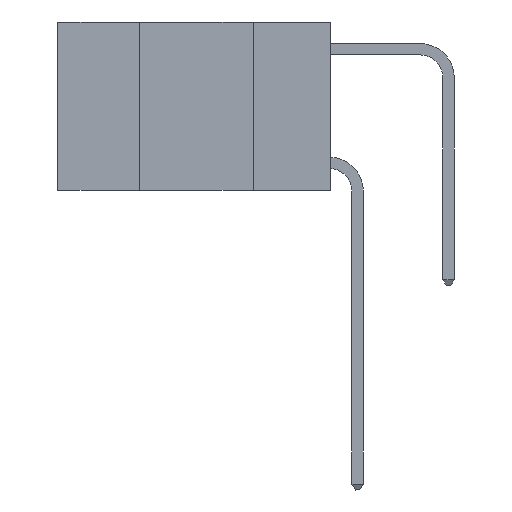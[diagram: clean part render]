
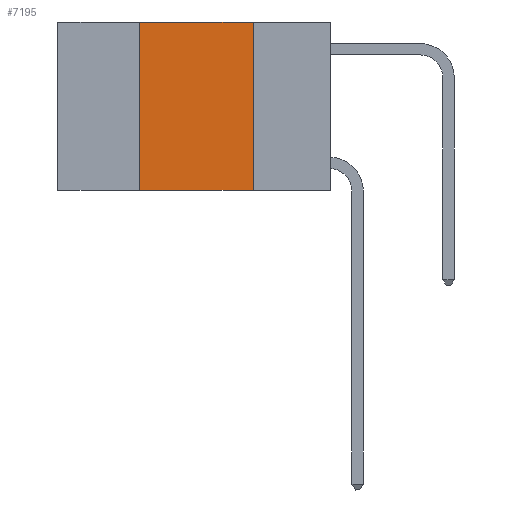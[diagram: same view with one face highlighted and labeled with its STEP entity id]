
A CAD part, left-side view. The second image highlights one B-rep face of the part: STEP entity #7195.
In plain terms, the highlighted planar face has unit normal (-1, 0, 0).
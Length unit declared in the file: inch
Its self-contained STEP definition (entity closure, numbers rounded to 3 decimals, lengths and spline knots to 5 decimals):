
#282 = CARTESIAN_POINT ( 'NONE',  ( 0., 0.6, 0. ) ) ;
#841 = VECTOR ( 'NONE', #5744, 39.37008 ) ;
#2904 = CARTESIAN_POINT ( 'NONE',  ( 0., 0.17, 0. ) ) ;
#2924 = CARTESIAN_POINT ( 'NONE',  ( 0., 0.6, 0. ) ) ;
#3123 = DIRECTION ( 'NONE',  ( 0., -1., 0. ) ) ;
#3323 = DIRECTION ( 'NONE',  ( 1., 0., 0. ) ) ;
#3525 = CARTESIAN_POINT ( 'NONE',  ( 0., 0.17, -0.37 ) ) ;
#3962 = CARTESIAN_POINT ( 'NONE',  ( 0., 0.42, -0.37 ) ) ;
#3967 = FACE_OUTER_BOUND ( 'NONE', #4237, .T. ) ;
#4157 = CARTESIAN_POINT ( 'NONE',  ( 0., 0.42, 0. ) ) ;
#4237 = EDGE_LOOP ( 'NONE', ( #6451, #6493, #6686, #6790 ) ) ;
#5332 = LINE ( 'NONE', #2904, #9069 ) ;
#5570 = LINE ( 'NONE', #11210, #841 ) ;
#5699 = VERTEX_POINT ( 'NONE', #8886 ) ;
#5744 = DIRECTION ( 'NONE',  ( 0., 0., 1. ) ) ;
#6025 = PLANE ( 'NONE',  #10023 ) ;
#6451 = ORIENTED_EDGE ( 'NONE', *, *, #10299, .F. ) ;
#6493 = ORIENTED_EDGE ( 'NONE', *, *, #6814, .F. ) ;
#6686 = ORIENTED_EDGE ( 'NONE', *, *, #11038, .F. ) ;
#6704 = CARTESIAN_POINT ( 'NONE',  ( 0., 0.6, -0.37 ) ) ;
#6790 = ORIENTED_EDGE ( 'NONE', *, *, #10481, .T. ) ;
#6791 = LINE ( 'NONE', #2924, #11077 ) ;
#6814 = EDGE_CURVE ( 'NONE', #8466, #5699, #6791, .T. ) ;
#7010 = VECTOR ( 'NONE', #3123, 39.37008 ) ;
#7195 = ADVANCED_FACE ( 'NONE', ( #3967 ), #6025, .F. ) ;
#7295 = LINE ( 'NONE', #6704, #7010 ) ;
#8466 = VERTEX_POINT ( 'NONE', #4157 ) ;
#8886 = CARTESIAN_POINT ( 'NONE',  ( 0., 0.17, 0. ) ) ;
#9069 = VECTOR ( 'NONE', #11934, 39.37008 ) ;
#9319 = VERTEX_POINT ( 'NONE', #3525 ) ;
#9689 = DIRECTION ( 'NONE',  ( 0., 0., -1. ) ) ;
#10023 = AXIS2_PLACEMENT_3D ( 'NONE', #282, #3323, #9689 ) ;
#10299 = EDGE_CURVE ( 'NONE', #5699, #9319, #5332, .T. ) ;
#10416 = VERTEX_POINT ( 'NONE', #3962 ) ;
#10481 = EDGE_CURVE ( 'NONE', #10416, #9319, #7295, .T. ) ;
#11038 = EDGE_CURVE ( 'NONE', #10416, #8466, #5570, .T. ) ;
#11077 = VECTOR ( 'NONE', #11115, 39.37008 ) ;
#11115 = DIRECTION ( 'NONE',  ( 0., -1., 0. ) ) ;
#11210 = CARTESIAN_POINT ( 'NONE',  ( 0., 0.42, 0. ) ) ;
#11934 = DIRECTION ( 'NONE',  ( 0., 0., -1. ) ) ;
